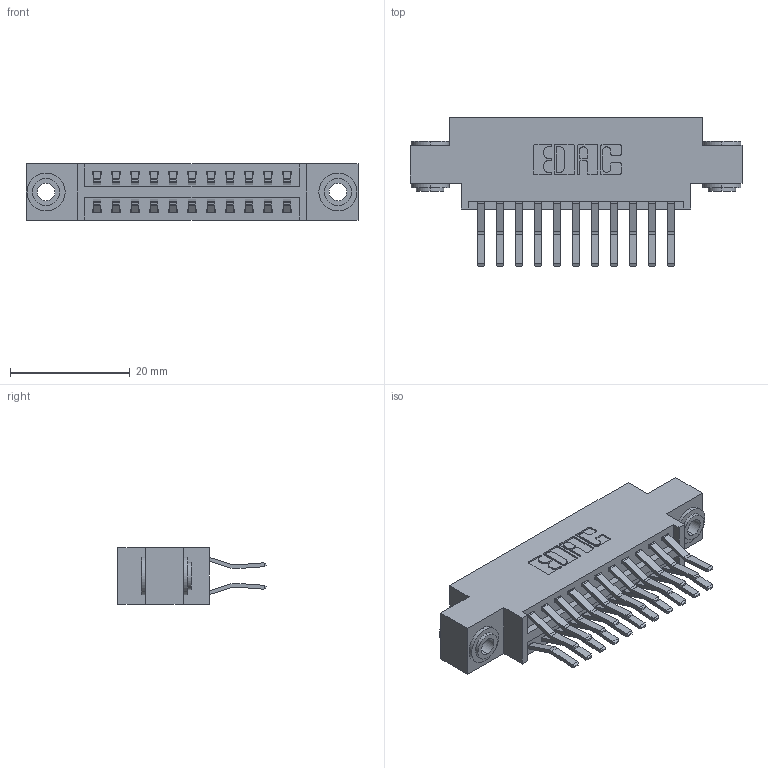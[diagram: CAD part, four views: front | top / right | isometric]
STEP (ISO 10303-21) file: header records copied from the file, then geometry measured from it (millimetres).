
FILE_DESCRIPTION (( 'STEP AP203' ), '1' );
FILE_NAME ('346-022-560-803.STEP', '2022-05-18T22:26:09', ( '' ), ( '' ), 'SwSTEP 2.0', 'SolidWorks 2020', '' );
FILE_SCHEMA (( 'CONFIG_CONTROL_DESIGN' ));
Length unit declared in the file: inch
Products named in the file (4): 346-022-560-803; 346 Part_0.170 Offset - 0.156 Dia-TH; 345-292-001_560 Tail; 345-250-002_345-250-002-102
Assembly tree (25 placements, depth 2):
  346-022-560-803
    346 Part_0.170 Offset - 0.156 Dia-TH
    345-292-001_560 Tail  x22
    345-250-002_345-250-002-102  x2
Bounding box: 55.5 x 24.78 x 9.4 mm (x, y, z)
Volume: 5162 mm3; surface area: 7421.3 mm2
Topology: 25 solids, 25 shells, 1366 faces, 3995 edges, 2630 vertices
Faces by surface type: plane 874, cylinder 484, cone 8
Entity records: 12638 total; most frequent: CARTESIAN_POINT 2109, ORIENTED_EDGE 2034, DIRECTION 1943, EDGE_CURVE 1017, LINE 813, VECTOR 813, VERTEX_POINT 674, AXIS2_PLACEMENT_3D 565
